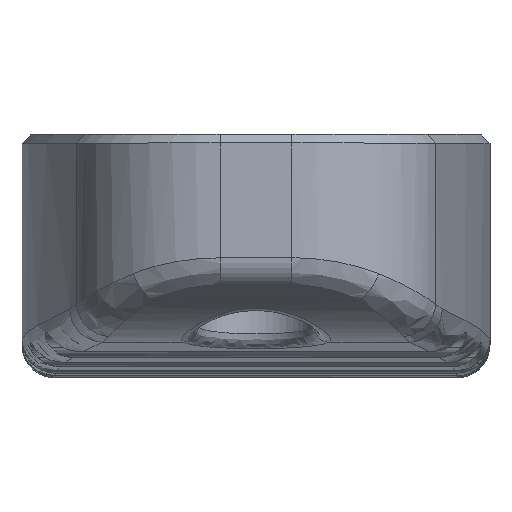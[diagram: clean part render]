
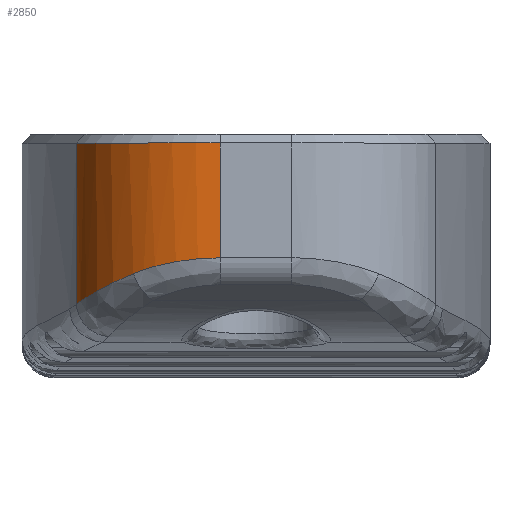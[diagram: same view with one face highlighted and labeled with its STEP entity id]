
A CAD part, top view. The second image highlights one B-rep face of the part: STEP entity #2850.
In plain terms, the highlighted cylindrical face has radius 10 mm (diameter 20 mm), a partial arc.
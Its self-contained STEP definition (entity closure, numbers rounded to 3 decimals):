
#222=LINE('',#6972,#376);
#223=LINE('',#6976,#377);
#376=VECTOR('',#3891,10.);
#377=VECTOR('',#3896,10.);
#475=CYLINDRICAL_SURFACE('',#3169,10.);
#590=B_SPLINE_CURVE_WITH_KNOTS('',3,(#6923,#6924,#6925,#6926,#6927),
 .UNSPECIFIED.,.F.,.F.,(4,1,4),(0.,0.247,0.577),
 .UNSPECIFIED.);
#742=FACE_OUTER_BOUND('',#928,.T.);
#928=EDGE_LOOP('',(#2534,#2535,#2536,#2537,#2538));
#975=ELLIPSE('',#3159,11.484,10.);
#1112=CIRCLE('',#3170,10.);
#1354=VERTEX_POINT('',#6884);
#1356=VERTEX_POINT('',#6921);
#1358=VERTEX_POINT('',#6949);
#1363=VERTEX_POINT('',#6971);
#1364=VERTEX_POINT('',#6975);
#1752=EDGE_CURVE('',#1356,#1354,#590,.T.);
#1754=EDGE_CURVE('',#1358,#1356,#975,.T.);
#1765=EDGE_CURVE('',#1363,#1354,#222,.T.);
#1767=EDGE_CURVE('',#1364,#1358,#223,.T.);
#1768=EDGE_CURVE('',#1363,#1364,#1112,.T.);
#2534=ORIENTED_EDGE('',*,*,#1752,.F.);
#2535=ORIENTED_EDGE('',*,*,#1754,.F.);
#2536=ORIENTED_EDGE('',*,*,#1767,.F.);
#2537=ORIENTED_EDGE('',*,*,#1768,.F.);
#2538=ORIENTED_EDGE('',*,*,#1765,.T.);
#2850=ADVANCED_FACE('',(#742),#475,.T.);
#3159=AXIS2_PLACEMENT_3D('',#6951,#3866,#3867);
#3169=AXIS2_PLACEMENT_3D('',#6974,#3894,#3895);
#3170=AXIS2_PLACEMENT_3D('',#6977,#3897,#3898);
#3866=DIRECTION('center_axis',(0.,-0.871,0.492));
#3867=DIRECTION('ref_axis',(0.,0.492,0.871));
#3891=DIRECTION('',(0.,-1.,0.));
#3894=DIRECTION('center_axis',(0.,-1.,0.));
#3895=DIRECTION('ref_axis',(-0.612,0.,0.791));
#3896=DIRECTION('',(0.,-1.,0.));
#3897=DIRECTION('center_axis',(0.,1.,0.));
#3898=DIRECTION('ref_axis',(-0.612,0.,0.791));
#6884=CARTESIAN_POINT('',(87.904,-715.44,125.108));
#6921=CARTESIAN_POINT('',(91.749,-713.392,130.728));
#6923=CARTESIAN_POINT('Ctrl Pts',(91.749,-713.392,130.728));
#6924=CARTESIAN_POINT('Ctrl Pts',(90.954,-713.714,130.157));
#6925=CARTESIAN_POINT('Ctrl Pts',(89.313,-714.508,128.57));
#6926=CARTESIAN_POINT('Ctrl Pts',(88.248,-715.177,126.441));
#6927=CARTESIAN_POINT('Ctrl Pts',(87.904,-715.44,125.108));
#6949=CARTESIAN_POINT('',(97.587,-712.33,132.609));
#6951=CARTESIAN_POINT('Origin',(97.587,-717.975,122.609));
#6971=CARTESIAN_POINT('',(87.904,-704.6,125.108));
#6972=CARTESIAN_POINT('',(87.904,-704.,125.108));
#6974=CARTESIAN_POINT('Origin',(97.587,-704.,122.609));
#6975=CARTESIAN_POINT('',(97.587,-704.6,132.609));
#6976=CARTESIAN_POINT('',(97.587,-704.,132.609));
#6977=CARTESIAN_POINT('Origin',(97.587,-704.6,122.609));
